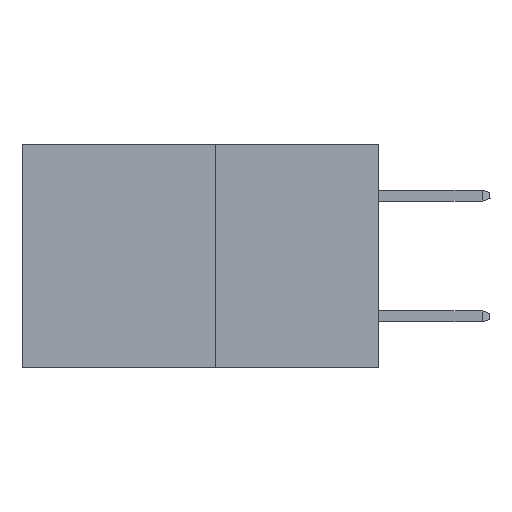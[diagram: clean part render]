
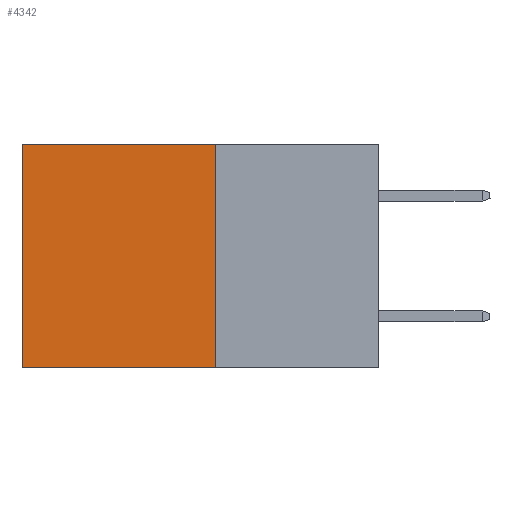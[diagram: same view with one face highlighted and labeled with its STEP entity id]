
A CAD part, left-side view. The second image highlights one B-rep face of the part: STEP entity #4342.
In plain terms, the highlighted planar face has unit normal (-1, 0, 0).
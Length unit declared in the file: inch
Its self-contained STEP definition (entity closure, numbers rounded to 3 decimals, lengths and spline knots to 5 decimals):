
#176 = ORIENTED_EDGE ( 'NONE', *, *, #12842, .T. ) ;
#468 = CARTESIAN_POINT ( 'NONE',  ( 0.277, 0.27, 0. ) ) ;
#813 = CARTESIAN_POINT ( 'NONE',  ( 0.277, 0.59, -0.37 ) ) ;
#1801 = VERTEX_POINT ( 'NONE', #468 ) ;
#1865 = EDGE_CURVE ( 'NONE', #14310, #6107, #15329, .T. ) ;
#2338 = AXIS2_PLACEMENT_3D ( 'NONE', #3539, #4947, #3609 ) ;
#3259 = CARTESIAN_POINT ( 'NONE',  ( 0.277, 0.59, -0.37 ) ) ;
#3285 = VECTOR ( 'NONE', #17710, 39.37008 ) ;
#3539 = CARTESIAN_POINT ( 'NONE',  ( 0.277, 0.27, -0.37 ) ) ;
#3609 = DIRECTION ( 'NONE',  ( 0., 0., -1. ) ) ;
#4271 = PLANE ( 'NONE',  #2338 ) ;
#4342 = ADVANCED_FACE ( 'NONE', ( #7038 ), #4271, .F. ) ;
#4795 = VECTOR ( 'NONE', #8845, 39.37008 ) ;
#4947 = DIRECTION ( 'NONE',  ( 1., 0., 0. ) ) ;
#6107 = VERTEX_POINT ( 'NONE', #813 ) ;
#6150 = EDGE_LOOP ( 'NONE', ( #176, #8367, #18026, #6336 ) ) ;
#6336 = ORIENTED_EDGE ( 'NONE', *, *, #10064, .T. ) ;
#7038 = FACE_OUTER_BOUND ( 'NONE', #6150, .T. ) ;
#7678 = VERTEX_POINT ( 'NONE', #17447 ) ;
#8367 = ORIENTED_EDGE ( 'NONE', *, *, #1865, .F. ) ;
#8845 = DIRECTION ( 'NONE',  ( 0., 1., 0. ) ) ;
#9060 = DIRECTION ( 'NONE',  ( 0., 0., -1. ) ) ;
#9155 = VECTOR ( 'NONE', #14019, 39.37008 ) ;
#10064 = EDGE_CURVE ( 'NONE', #1801, #7678, #16875, .T. ) ;
#10722 = LINE ( 'NONE', #3259, #19162 ) ;
#12842 = EDGE_CURVE ( 'NONE', #7678, #6107, #10722, .T. ) ;
#13250 = CARTESIAN_POINT ( 'NONE',  ( 0.277, 0.27, -0.37 ) ) ;
#14019 = DIRECTION ( 'NONE',  ( 0., 0., -1. ) ) ;
#14310 = VERTEX_POINT ( 'NONE', #13250 ) ;
#15273 = EDGE_CURVE ( 'NONE', #1801, #14310, #17625, .T. ) ;
#15329 = LINE ( 'NONE', #17646, #3285 ) ;
#16875 = LINE ( 'NONE', #20171, #4795 ) ;
#17447 = CARTESIAN_POINT ( 'NONE',  ( 0.277, 0.59, 0. ) ) ;
#17625 = LINE ( 'NONE', #17925, #9155 ) ;
#17646 = CARTESIAN_POINT ( 'NONE',  ( 0.277, 0.27, -0.37 ) ) ;
#17710 = DIRECTION ( 'NONE',  ( 0., 1., 0. ) ) ;
#17925 = CARTESIAN_POINT ( 'NONE',  ( 0.277, 0.27, -0.37 ) ) ;
#18026 = ORIENTED_EDGE ( 'NONE', *, *, #15273, .F. ) ;
#19162 = VECTOR ( 'NONE', #9060, 39.37008 ) ;
#20171 = CARTESIAN_POINT ( 'NONE',  ( 0.277, 0.27, 0. ) ) ;
